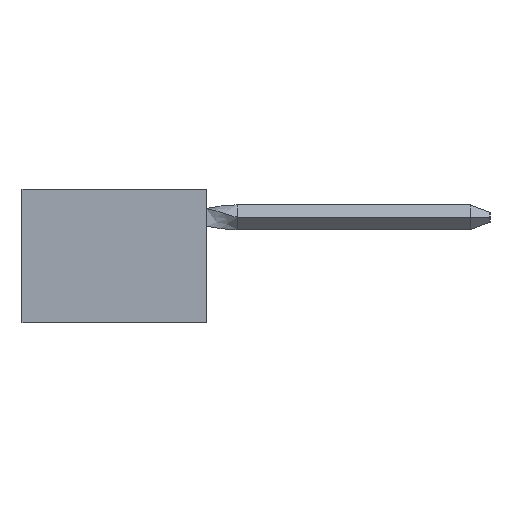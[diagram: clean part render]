
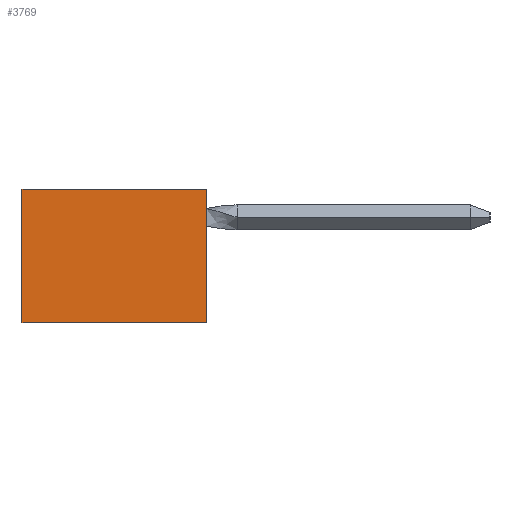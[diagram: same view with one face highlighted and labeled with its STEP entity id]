
A CAD part, left-side view. The second image highlights one B-rep face of the part: STEP entity #3769.
In plain terms, the highlighted planar face has unit normal (-1, 0, 0).
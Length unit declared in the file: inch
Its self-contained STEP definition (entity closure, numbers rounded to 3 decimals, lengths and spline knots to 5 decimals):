
#1228 = VECTOR ( 'NONE', #30179, 39.37008 ) ;
#1641 = DIRECTION ( 'NONE',  ( 0., 0., -1. ) ) ;
#2139 = VECTOR ( 'NONE', #40041, 39.37008 ) ;
#2997 = VECTOR ( 'NONE', #15669, 39.37008 ) ;
#3769 = ADVANCED_FACE ( 'NONE', ( #12467 ), #32309, .F. ) ;
#4147 = CARTESIAN_POINT ( 'NONE',  ( 0.298, 0.473, 0. ) ) ;
#4588 = VERTEX_POINT ( 'NONE', #4147 ) ;
#4991 = CARTESIAN_POINT ( 'NONE',  ( 0.298, 0., 0. ) ) ;
#9886 = EDGE_CURVE ( 'NONE', #4588, #14314, #26257, .T. ) ;
#10435 = CARTESIAN_POINT ( 'NONE',  ( 0.298, 0.473, -0.343 ) ) ;
#11411 = DIRECTION ( 'NONE',  ( 1., 0., 0. ) ) ;
#11799 = VERTEX_POINT ( 'NONE', #26771 ) ;
#12467 = FACE_OUTER_BOUND ( 'NONE', #14784, .T. ) ;
#12827 = CARTESIAN_POINT ( 'NONE',  ( 0.298, 0.473, -0.343 ) ) ;
#14314 = VERTEX_POINT ( 'NONE', #10435 ) ;
#14784 = EDGE_LOOP ( 'NONE', ( #42826, #29731, #35256, #19823 ) ) ;
#15669 = DIRECTION ( 'NONE',  ( 0., 0., 1. ) ) ;
#16291 = AXIS2_PLACEMENT_3D ( 'NONE', #22155, #11411, #1641 ) ;
#17057 = CARTESIAN_POINT ( 'NONE',  ( 0.298, -0.027, 0. ) ) ;
#17886 = LINE ( 'NONE', #35942, #2997 ) ;
#19823 = ORIENTED_EDGE ( 'NONE', *, *, #39395, .F. ) ;
#21612 = VERTEX_POINT ( 'NONE', #4991 ) ;
#22155 = CARTESIAN_POINT ( 'NONE',  ( 0.298, -0.027, 0. ) ) ;
#22241 = EDGE_CURVE ( 'NONE', #11799, #21612, #17886, .T. ) ;
#25535 = LINE ( 'NONE', #17057, #30842 ) ;
#26257 = LINE ( 'NONE', #40356, #1228 ) ;
#26771 = CARTESIAN_POINT ( 'NONE',  ( 0.298, 0., -0.343 ) ) ;
#27077 = DIRECTION ( 'NONE',  ( 0., 1., 0. ) ) ;
#29731 = ORIENTED_EDGE ( 'NONE', *, *, #30027, .T. ) ;
#30027 = EDGE_CURVE ( 'NONE', #21612, #4588, #25535, .T. ) ;
#30179 = DIRECTION ( 'NONE',  ( 0., 0., -1. ) ) ;
#30842 = VECTOR ( 'NONE', #27077, 39.37008 ) ;
#32309 = PLANE ( 'NONE',  #16291 ) ;
#33043 = LINE ( 'NONE', #12827, #2139 ) ;
#35256 = ORIENTED_EDGE ( 'NONE', *, *, #9886, .T. ) ;
#35942 = CARTESIAN_POINT ( 'NONE',  ( 0.298, 0., -0.343 ) ) ;
#39395 = EDGE_CURVE ( 'NONE', #11799, #14314, #33043, .T. ) ;
#40041 = DIRECTION ( 'NONE',  ( 0., 1., 0. ) ) ;
#40356 = CARTESIAN_POINT ( 'NONE',  ( 0.298, 0.473, 0. ) ) ;
#42826 = ORIENTED_EDGE ( 'NONE', *, *, #22241, .T. ) ;
